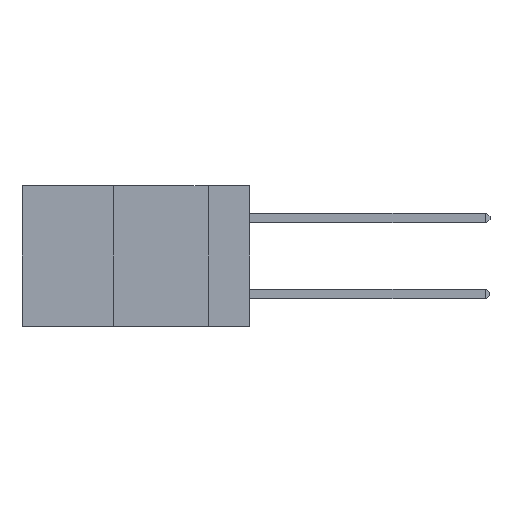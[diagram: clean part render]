
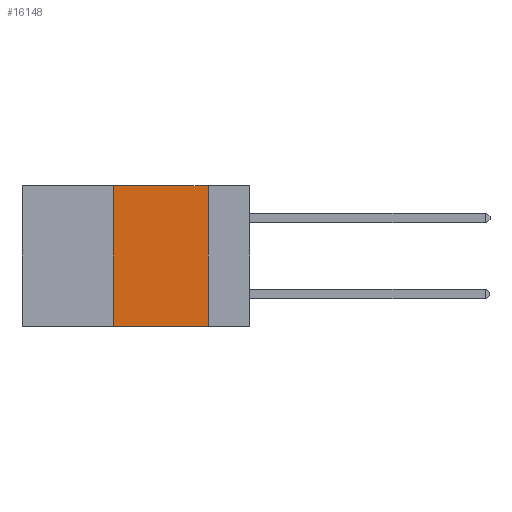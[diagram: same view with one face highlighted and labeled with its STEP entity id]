
A CAD part, left-side view. The second image highlights one B-rep face of the part: STEP entity #16148.
In plain terms, the highlighted planar face has unit normal (-1, 0, 0).
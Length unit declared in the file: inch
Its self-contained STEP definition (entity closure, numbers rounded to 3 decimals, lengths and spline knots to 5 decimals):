
#362 = DIRECTION ( 'NONE',  ( 0., -1., 0. ) ) ;
#1092 = VECTOR ( 'NONE', #18017, 39.37008 ) ;
#1502 = CARTESIAN_POINT ( 'NONE',  ( 0., 0.11, 0. ) ) ;
#1545 = EDGE_LOOP ( 'NONE', ( #20868, #9514, #10034, #3197 ) ) ;
#1692 = VERTEX_POINT ( 'NONE', #8824 ) ;
#1888 = AXIS2_PLACEMENT_3D ( 'NONE', #5984, #2619, #14217 ) ;
#2119 = EDGE_CURVE ( 'NONE', #9214, #1692, #10054, .T. ) ;
#2619 = DIRECTION ( 'NONE',  ( 1., 0., 0. ) ) ;
#2792 = VERTEX_POINT ( 'NONE', #15071 ) ;
#3197 = ORIENTED_EDGE ( 'NONE', *, *, #8593, .T. ) ;
#3304 = VECTOR ( 'NONE', #17069, 39.37008 ) ;
#5059 = LINE ( 'NONE', #7460, #8950 ) ;
#5984 = CARTESIAN_POINT ( 'NONE',  ( 0., 0.6, 0. ) ) ;
#6563 = CARTESIAN_POINT ( 'NONE',  ( 0., 0.36, -0.37 ) ) ;
#7460 = CARTESIAN_POINT ( 'NONE',  ( 0., 0.6, 0. ) ) ;
#7927 = FACE_OUTER_BOUND ( 'NONE', #1545, .T. ) ;
#8331 = LINE ( 'NONE', #10447, #16486 ) ;
#8593 = EDGE_CURVE ( 'NONE', #20414, #1692, #8331, .T. ) ;
#8824 = CARTESIAN_POINT ( 'NONE',  ( 0., 0.11, -0.37 ) ) ;
#8950 = VECTOR ( 'NONE', #15604, 39.37008 ) ;
#9214 = VERTEX_POINT ( 'NONE', #15331 ) ;
#9514 = ORIENTED_EDGE ( 'NONE', *, *, #16054, .F. ) ;
#10034 = ORIENTED_EDGE ( 'NONE', *, *, #19459, .F. ) ;
#10054 = LINE ( 'NONE', #1502, #1092 ) ;
#10447 = CARTESIAN_POINT ( 'NONE',  ( 0., 0.6, -0.37 ) ) ;
#12602 = PLANE ( 'NONE',  #1888 ) ;
#13155 = LINE ( 'NONE', #13870, #3304 ) ;
#13870 = CARTESIAN_POINT ( 'NONE',  ( 0., 0.36, 0. ) ) ;
#14217 = DIRECTION ( 'NONE',  ( 0., 0., -1. ) ) ;
#15071 = CARTESIAN_POINT ( 'NONE',  ( 0., 0.36, 0. ) ) ;
#15331 = CARTESIAN_POINT ( 'NONE',  ( 0., 0.11, 0. ) ) ;
#15604 = DIRECTION ( 'NONE',  ( 0., -1., 0. ) ) ;
#16054 = EDGE_CURVE ( 'NONE', #2792, #9214, #5059, .T. ) ;
#16148 = ADVANCED_FACE ( 'NONE', ( #7927 ), #12602, .F. ) ;
#16486 = VECTOR ( 'NONE', #362, 39.37008 ) ;
#17069 = DIRECTION ( 'NONE',  ( 0., 0., 1. ) ) ;
#18017 = DIRECTION ( 'NONE',  ( 0., 0., -1. ) ) ;
#19459 = EDGE_CURVE ( 'NONE', #20414, #2792, #13155, .T. ) ;
#20414 = VERTEX_POINT ( 'NONE', #6563 ) ;
#20868 = ORIENTED_EDGE ( 'NONE', *, *, #2119, .F. ) ;
